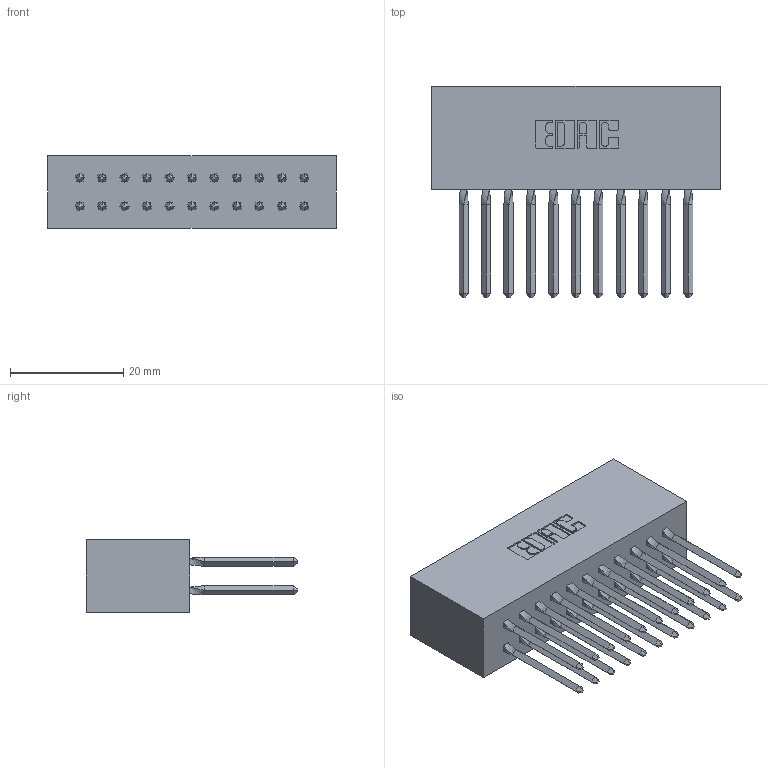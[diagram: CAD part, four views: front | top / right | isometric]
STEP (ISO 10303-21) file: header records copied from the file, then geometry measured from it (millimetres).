
FILE_DESCRIPTION (( 'STEP AP203' ), '1' );
FILE_NAME ('317-022-542-801.STEP', '2020-02-27T17:26:37', ( '' ), ( '' ), 'SwSTEP 2.0', 'SolidWorks 2016', '' );
FILE_SCHEMA (( 'CONFIG_CONTROL_DESIGN' ));
Length unit declared in the file: inch
Products named in the file (3): 317-290-003_542; 317 Part_Lugless; 317-022-542-801
Assembly tree (23 placements, depth 2):
  317-022-542-801
    317 Part_Lugless
    317-290-003_542  x22
Bounding box: 50.8 x 37.34 x 12.7 mm (x, y, z)
Volume: 9068.9 mm3; surface area: 11793.2 mm2
Topology: 23 solids, 23 shells, 1344 faces, 3759 edges, 2402 vertices
Faces by surface type: plane 1062, cylinder 194, bspline 88
Entity records: 18833 total; most frequent: CARTESIAN_POINT 3529, ORIENTED_EDGE 3192, DIRECTION 2732, EDGE_CURVE 1596, VECTOR 1434, LINE 1434, VERTEX_POINT 1058, AXIS2_PLACEMENT_3D 649
